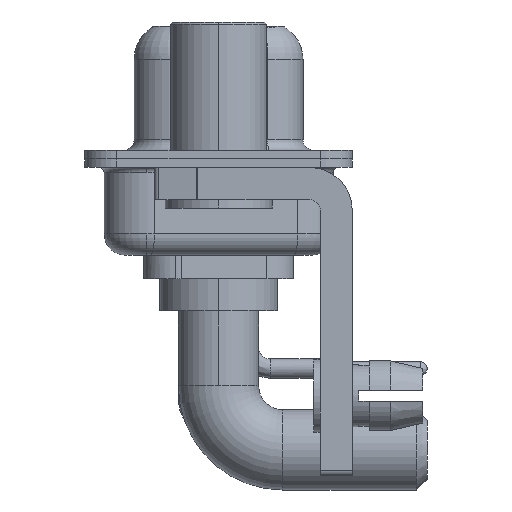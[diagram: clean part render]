
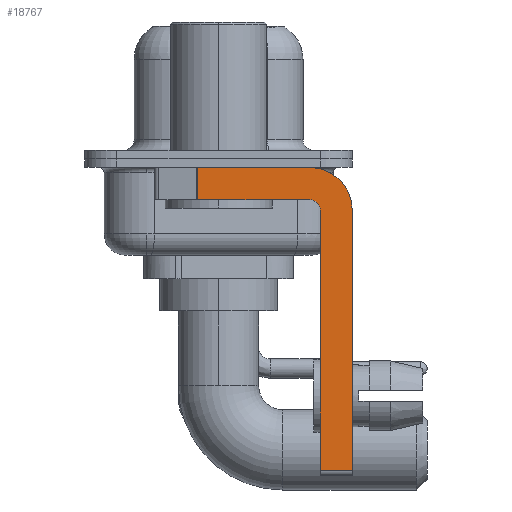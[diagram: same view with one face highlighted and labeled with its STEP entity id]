
A CAD part, left-side view. The second image highlights one B-rep face of the part: STEP entity #18767.
In plain terms, the highlighted planar face has unit normal (-1, 0, 0).
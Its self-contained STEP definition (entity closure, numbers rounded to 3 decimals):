
#436 = DIRECTION ( 'NONE',  ( 0., 1., 0. ) ) ;
#492 = DIRECTION ( 'NONE',  ( -1., 0., 0. ) ) ;
#1085 = DIRECTION ( 'NONE',  ( 0., 0., 1. ) ) ;
#1184 = VERTEX_POINT ( 'NONE', #14165 ) ;
#1436 = EDGE_LOOP ( 'NONE', ( #10776, #9390, #20988, #17458, #11431, #2010, #1470, #16121 ) ) ;
#1470 = ORIENTED_EDGE ( 'NONE', *, *, #9552, .F. ) ;
#1557 = LINE ( 'NONE', #9427, #7755 ) ;
#2010 = ORIENTED_EDGE ( 'NONE', *, *, #4455, .T. ) ;
#2434 = AXIS2_PLACEMENT_3D ( 'NONE', #13314, #3411, #3307 ) ;
#2867 = EDGE_CURVE ( 'NONE', #6288, #11117, #13638, .T. ) ;
#3193 = DIRECTION ( 'NONE',  ( 1., 0., 0. ) ) ;
#3307 = DIRECTION ( 'NONE',  ( 0., 0., -1. ) ) ;
#3325 = VERTEX_POINT ( 'NONE', #10424 ) ;
#3411 = DIRECTION ( 'NONE',  ( 1., 0., 0. ) ) ;
#4281 = VECTOR ( 'NONE', #1085, 1000. ) ;
#4455 = EDGE_CURVE ( 'NONE', #1184, #8827, #8652, .T. ) ;
#4459 = CARTESIAN_POINT ( 'NONE',  ( -2.9, -6.25, -14.55 ) ) ;
#4570 = EDGE_CURVE ( 'NONE', #1184, #3325, #18862, .T. ) ;
#4905 = FACE_OUTER_BOUND ( 'NONE', #1436, .T. ) ;
#5200 = CARTESIAN_POINT ( 'NONE',  ( -2.9, -4.25, -2.4 ) ) ;
#5283 = CARTESIAN_POINT ( 'NONE',  ( -2.9, 0.978, -0.4 ) ) ;
#5987 = LINE ( 'NONE', #7778, #10845 ) ;
#6265 = VECTOR ( 'NONE', #436, 1000. ) ;
#6288 = VERTEX_POINT ( 'NONE', #15443 ) ;
#7301 = DIRECTION ( 'NONE',  ( 0., -1., 0. ) ) ;
#7557 = VERTEX_POINT ( 'NONE', #13854 ) ;
#7677 = DIRECTION ( 'NONE',  ( 0., -1., 0. ) ) ;
#7755 = VECTOR ( 'NONE', #16033, 1000. ) ;
#7778 = CARTESIAN_POINT ( 'NONE',  ( -2.9, -6.25, -2.4 ) ) ;
#7858 = EDGE_CURVE ( 'NONE', #7557, #13078, #16555, .T. ) ;
#8515 = CARTESIAN_POINT ( 'NONE',  ( -2.9, -4.25, -1.9 ) ) ;
#8542 = CARTESIAN_POINT ( 'NONE',  ( -2.9, -4.25, -14.55 ) ) ;
#8652 = LINE ( 'NONE', #8542, #16859 ) ;
#8762 = CARTESIAN_POINT ( 'NONE',  ( -2.9, 0.978, -1.9 ) ) ;
#8827 = VERTEX_POINT ( 'NONE', #4459 ) ;
#9211 = CIRCLE ( 'NONE', #19406, 0.5 ) ;
#9223 = EDGE_CURVE ( 'NONE', #14256, #11117, #1557, .T. ) ;
#9390 = ORIENTED_EDGE ( 'NONE', *, *, #9223, .T. ) ;
#9427 = CARTESIAN_POINT ( 'NONE',  ( -2.9, 0.978, -1.9 ) ) ;
#9552 = EDGE_CURVE ( 'NONE', #13078, #8827, #5987, .T. ) ;
#10424 = CARTESIAN_POINT ( 'NONE',  ( -2.9, -4.75, -2.4 ) ) ;
#10615 = VECTOR ( 'NONE', #7301, 1000. ) ;
#10776 = ORIENTED_EDGE ( 'NONE', *, *, #14482, .F. ) ;
#10845 = VECTOR ( 'NONE', #20561, 1000. ) ;
#11117 = VERTEX_POINT ( 'NONE', #8762 ) ;
#11407 = PLANE ( 'NONE',  #2434 ) ;
#11431 = ORIENTED_EDGE ( 'NONE', *, *, #4570, .F. ) ;
#11466 = AXIS2_PLACEMENT_3D ( 'NONE', #5200, #3193, #17859 ) ;
#12443 = CARTESIAN_POINT ( 'NONE',  ( -2.9, -6.25, -2.4 ) ) ;
#12593 = CARTESIAN_POINT ( 'NONE',  ( -2.9, -4.75, -14.8 ) ) ;
#13078 = VERTEX_POINT ( 'NONE', #12443 ) ;
#13314 = CARTESIAN_POINT ( 'NONE',  ( -2.9, -4.25, -2.4 ) ) ;
#13448 = EDGE_CURVE ( 'NONE', #3325, #6288, #9211, .T. ) ;
#13638 = LINE ( 'NONE', #8515, #6265 ) ;
#13854 = CARTESIAN_POINT ( 'NONE',  ( -2.9, -4.25, -0.4 ) ) ;
#14165 = CARTESIAN_POINT ( 'NONE',  ( -2.9, -4.75, -14.55 ) ) ;
#14256 = VERTEX_POINT ( 'NONE', #5283 ) ;
#14482 = EDGE_CURVE ( 'NONE', #14256, #7557, #18781, .T. ) ;
#14734 = DIRECTION ( 'NONE',  ( 0., 0., 1. ) ) ;
#15443 = CARTESIAN_POINT ( 'NONE',  ( -2.9, -4.25, -1.9 ) ) ;
#16033 = DIRECTION ( 'NONE',  ( 0., 0., -1. ) ) ;
#16121 = ORIENTED_EDGE ( 'NONE', *, *, #7858, .F. ) ;
#16547 = CARTESIAN_POINT ( 'NONE',  ( -2.9, -4.25, -2.4 ) ) ;
#16555 = CIRCLE ( 'NONE', #11466, 2. ) ;
#16859 = VECTOR ( 'NONE', #7677, 1000. ) ;
#17191 = CARTESIAN_POINT ( 'NONE',  ( -2.9, 3., -0.4 ) ) ;
#17458 = ORIENTED_EDGE ( 'NONE', *, *, #13448, .F. ) ;
#17859 = DIRECTION ( 'NONE',  ( 0., 0., -1. ) ) ;
#18767 = ADVANCED_FACE ( 'NONE', ( #4905 ), #11407, .F. ) ;
#18781 = LINE ( 'NONE', #17191, #10615 ) ;
#18862 = LINE ( 'NONE', #12593, #4281 ) ;
#19406 = AXIS2_PLACEMENT_3D ( 'NONE', #16547, #492, #14734 ) ;
#20561 = DIRECTION ( 'NONE',  ( 0., 0., -1. ) ) ;
#20988 = ORIENTED_EDGE ( 'NONE', *, *, #2867, .F. ) ;
